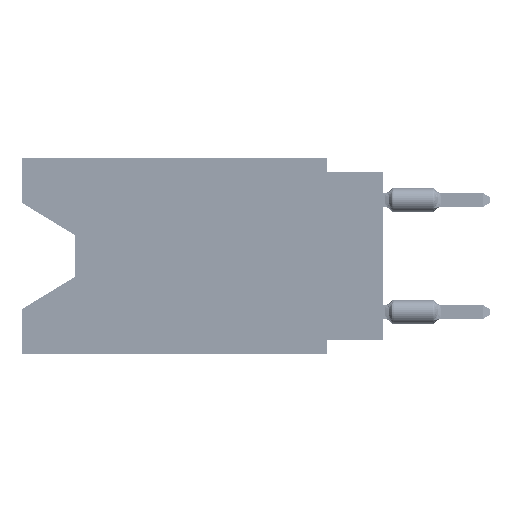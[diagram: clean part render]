
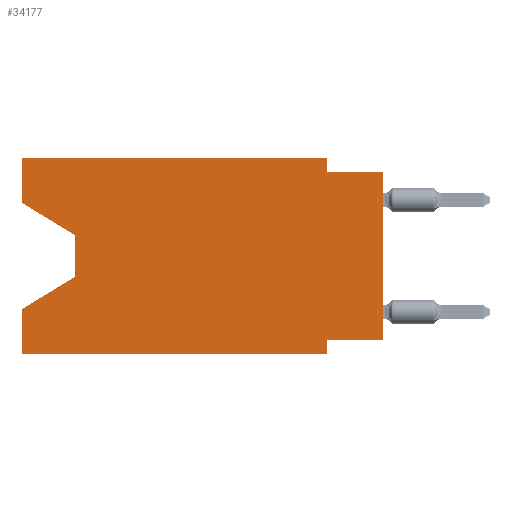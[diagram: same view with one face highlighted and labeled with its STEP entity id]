
A CAD part, left-side view. The second image highlights one B-rep face of the part: STEP entity #34177.
In plain terms, the highlighted planar face has unit normal (-1, 0, 0).
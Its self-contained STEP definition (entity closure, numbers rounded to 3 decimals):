
#2908 = VECTOR ( 'NONE', #95545, 1000. ) ;
#4387 = EDGE_CURVE ( 'NONE', #27407, #40838, #99157, .T. ) ;
#4903 = VERTEX_POINT ( 'NONE', #75548 ) ;
#5578 = DIRECTION ( 'NONE',  ( 0., -1., 0. ) ) ;
#5663 = VECTOR ( 'NONE', #44309, 1000. ) ;
#6816 = CARTESIAN_POINT ( 'NONE',  ( 0., 16.383, -6.852 ) ) ;
#7006 = ORIENTED_EDGE ( 'NONE', *, *, #24586, .T. ) ;
#7075 = DIRECTION ( 'NONE',  ( 0., 0., -1. ) ) ;
#8519 = LINE ( 'NONE', #73767, #83825 ) ;
#9525 = CARTESIAN_POINT ( 'NONE',  ( 0., 2.54, -0.635 ) ) ;
#10647 = VECTOR ( 'NONE', #94173, 1000. ) ;
#12467 = LINE ( 'NONE', #58957, #5663 ) ;
#12518 = VECTOR ( 'NONE', #18026, 1000. ) ;
#12730 = CARTESIAN_POINT ( 'NONE',  ( 0., 16.383, 0. ) ) ;
#14506 = EDGE_CURVE ( 'NONE', #96714, #27407, #8519, .T. ) ;
#15878 = EDGE_CURVE ( 'NONE', #83076, #39341, #40517, .T. ) ;
#17486 = CARTESIAN_POINT ( 'NONE',  ( 0., 16.383, 0. ) ) ;
#18026 = DIRECTION ( 'NONE',  ( 0., -1., 0. ) ) ;
#18618 = CARTESIAN_POINT ( 'NONE',  ( 0., 13.97, -5.385 ) ) ;
#19156 = DIRECTION ( 'NONE',  ( 0., 0., -1. ) ) ;
#20188 = ORIENTED_EDGE ( 'NONE', *, *, #43302, .F. ) ;
#21144 = VERTEX_POINT ( 'NONE', #9525 ) ;
#22151 = CARTESIAN_POINT ( 'NONE',  ( 0., 16.383, -2.038 ) ) ;
#22486 = EDGE_CURVE ( 'NONE', #4903, #88690, #26368, .T. ) ;
#24183 = CARTESIAN_POINT ( 'NONE',  ( 0., 2.54, 0. ) ) ;
#24586 = EDGE_CURVE ( 'NONE', #54272, #44017, #101588, .T. ) ;
#25693 = ORIENTED_EDGE ( 'NONE', *, *, #27617, .T. ) ;
#26368 = LINE ( 'NONE', #17486, #48265 ) ;
#27000 = PLANE ( 'NONE',  #49842 ) ;
#27407 = VERTEX_POINT ( 'NONE', #36272 ) ;
#27617 = EDGE_CURVE ( 'NONE', #81159, #54272, #62332, .T. ) ;
#27635 = CARTESIAN_POINT ( 'NONE',  ( 0., 2.54, -8.89 ) ) ;
#28030 = EDGE_CURVE ( 'NONE', #21144, #44791, #12467, .T. ) ;
#28161 = VECTOR ( 'NONE', #82472, 1000. ) ;
#29022 = ORIENTED_EDGE ( 'NONE', *, *, #99690, .F. ) ;
#30011 = VECTOR ( 'NONE', #7075, 1000. ) ;
#31847 = LINE ( 'NONE', #63695, #2908 ) ;
#32466 = EDGE_CURVE ( 'NONE', #96714, #44791, #31847, .T. ) ;
#34177 = ADVANCED_FACE ( 'NONE', ( #98515 ), #27000, .F. ) ;
#34609 = ORIENTED_EDGE ( 'NONE', *, *, #22486, .F. ) ;
#34789 = DIRECTION ( 'NONE',  ( 0., 0.855, -0.519 ) ) ;
#36272 = CARTESIAN_POINT ( 'NONE',  ( 0., 2.54, -8.255 ) ) ;
#38284 = LINE ( 'NONE', #70137, #80042 ) ;
#39341 = VERTEX_POINT ( 'NONE', #24183 ) ;
#40517 = LINE ( 'NONE', #53357, #12518 ) ;
#40838 = VERTEX_POINT ( 'NONE', #73422 ) ;
#41803 = ORIENTED_EDGE ( 'NONE', *, *, #79257, .T. ) ;
#43302 = EDGE_CURVE ( 'NONE', #81159, #83076, #95541, .T. ) ;
#43884 = ORIENTED_EDGE ( 'NONE', *, *, #55137, .T. ) ;
#44017 = VERTEX_POINT ( 'NONE', #85281 ) ;
#44309 = DIRECTION ( 'NONE',  ( 0., -1., 0. ) ) ;
#44791 = VERTEX_POINT ( 'NONE', #80410 ) ;
#48265 = VECTOR ( 'NONE', #96876, 1000. ) ;
#48599 = VECTOR ( 'NONE', #73065, 1000. ) ;
#49624 = ORIENTED_EDGE ( 'NONE', *, *, #32466, .T. ) ;
#49842 = AXIS2_PLACEMENT_3D ( 'NONE', #75535, #90682, #19156 ) ;
#53357 = CARTESIAN_POINT ( 'NONE',  ( 0., 16.383, 0. ) ) ;
#54272 = VERTEX_POINT ( 'NONE', #91414 ) ;
#55137 = EDGE_CURVE ( 'NONE', #44017, #88690, #91163, .T. ) ;
#57560 = DIRECTION ( 'NONE',  ( 0., 1., 0. ) ) ;
#58957 = CARTESIAN_POINT ( 'NONE',  ( 0., 0., -0.635 ) ) ;
#62332 = LINE ( 'NONE', #22151, #10647 ) ;
#63695 = CARTESIAN_POINT ( 'NONE',  ( 0., 0., 0. ) ) ;
#70137 = CARTESIAN_POINT ( 'NONE',  ( 0., 2.54, 0. ) ) ;
#71290 = CARTESIAN_POINT ( 'NONE',  ( 0., 13.97, -3.505 ) ) ;
#72043 = CARTESIAN_POINT ( 'NONE',  ( 0., 16.383, 0. ) ) ;
#73065 = DIRECTION ( 'NONE',  ( 0., 0., 1. ) ) ;
#73422 = CARTESIAN_POINT ( 'NONE',  ( 0., 2.54, -8.89 ) ) ;
#73767 = CARTESIAN_POINT ( 'NONE',  ( 0., 0., -8.255 ) ) ;
#75535 = CARTESIAN_POINT ( 'NONE',  ( 0., 16.383, 0. ) ) ;
#75548 = CARTESIAN_POINT ( 'NONE',  ( 0., 16.383, -8.89 ) ) ;
#75615 = VECTOR ( 'NONE', #5578, 1000. ) ;
#77103 = LINE ( 'NONE', #77606, #75615 ) ;
#77329 = ORIENTED_EDGE ( 'NONE', *, *, #28030, .F. ) ;
#77606 = CARTESIAN_POINT ( 'NONE',  ( 0., 16.383, -8.89 ) ) ;
#79257 = EDGE_CURVE ( 'NONE', #4903, #40838, #77103, .T. ) ;
#79961 = ORIENTED_EDGE ( 'NONE', *, *, #4387, .F. ) ;
#80042 = VECTOR ( 'NONE', #86827, 1000. ) ;
#80226 = ORIENTED_EDGE ( 'NONE', *, *, #15878, .F. ) ;
#80410 = CARTESIAN_POINT ( 'NONE',  ( 0., 0., -0.635 ) ) ;
#80713 = ORIENTED_EDGE ( 'NONE', *, *, #14506, .F. ) ;
#81159 = VERTEX_POINT ( 'NONE', #94361 ) ;
#82472 = DIRECTION ( 'NONE',  ( 0., 0., -1. ) ) ;
#83076 = VERTEX_POINT ( 'NONE', #12730 ) ;
#83327 = CARTESIAN_POINT ( 'NONE',  ( 0., 0., -8.255 ) ) ;
#83825 = VECTOR ( 'NONE', #57560, 1000. ) ;
#84705 = VECTOR ( 'NONE', #34789, 1000. ) ;
#85281 = CARTESIAN_POINT ( 'NONE',  ( 0., 13.97, -5.385 ) ) ;
#86827 = DIRECTION ( 'NONE',  ( 0., 0., -1. ) ) ;
#87755 = EDGE_LOOP ( 'NONE', ( #25693, #7006, #43884, #34609, #41803, #79961, #80713, #49624, #77329, #29022, #80226, #20188 ) ) ;
#88690 = VERTEX_POINT ( 'NONE', #6816 ) ;
#90682 = DIRECTION ( 'NONE',  ( 1., 0., 0. ) ) ;
#91163 = LINE ( 'NONE', #18618, #84705 ) ;
#91414 = CARTESIAN_POINT ( 'NONE',  ( 0., 13.97, -3.505 ) ) ;
#94173 = DIRECTION ( 'NONE',  ( 0., -0.855, -0.519 ) ) ;
#94361 = CARTESIAN_POINT ( 'NONE',  ( 0., 16.383, -2.038 ) ) ;
#95541 = LINE ( 'NONE', #72043, #48599 ) ;
#95545 = DIRECTION ( 'NONE',  ( 0., 0., 1. ) ) ;
#96714 = VERTEX_POINT ( 'NONE', #83327 ) ;
#96876 = DIRECTION ( 'NONE',  ( 0., 0., 1. ) ) ;
#98515 = FACE_OUTER_BOUND ( 'NONE', #87755, .T. ) ;
#99157 = LINE ( 'NONE', #27635, #28161 ) ;
#99690 = EDGE_CURVE ( 'NONE', #39341, #21144, #38284, .T. ) ;
#101588 = LINE ( 'NONE', #71290, #30011 ) ;
